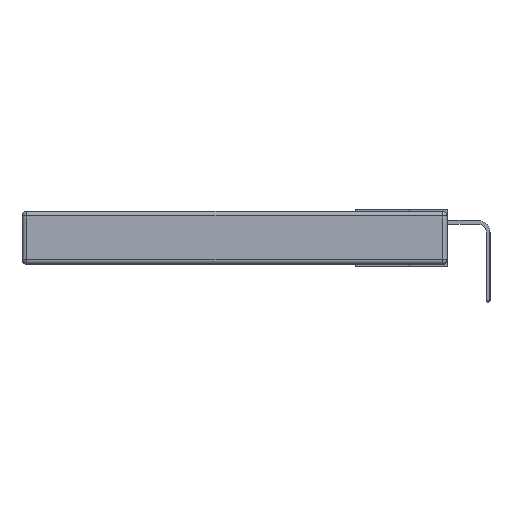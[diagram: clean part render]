
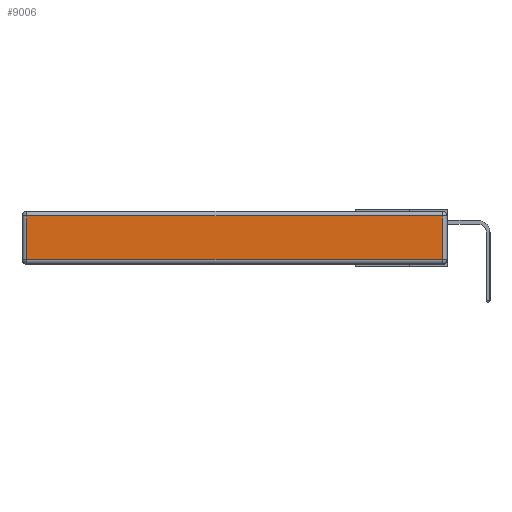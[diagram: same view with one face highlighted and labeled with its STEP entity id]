
A CAD part, left-side view. The second image highlights one B-rep face of the part: STEP entity #9006.
In plain terms, the highlighted planar face has unit normal (-1, 0, 0).
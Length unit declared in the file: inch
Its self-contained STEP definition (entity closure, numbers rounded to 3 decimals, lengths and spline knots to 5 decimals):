
#140 = PLANE ( 'NONE',  #7943 ) ;
#182 = DIRECTION ( 'NONE',  ( 0., 0., -1. ) ) ;
#898 = DIRECTION ( 'NONE',  ( 0., 1., 0. ) ) ;
#986 = VERTEX_POINT ( 'NONE', #5467 ) ;
#1932 = VECTOR ( 'NONE', #182, 39.37008 ) ;
#2548 = ORIENTED_EDGE ( 'NONE', *, *, #2623, .T. ) ;
#2623 = EDGE_CURVE ( 'NONE', #986, #3950, #15878, .T. ) ;
#2665 = CARTESIAN_POINT ( 'NONE',  ( 0., 2.72, -0.03 ) ) ;
#2863 = CARTESIAN_POINT ( 'NONE',  ( 0., 0., -0.343 ) ) ;
#3231 = FACE_OUTER_BOUND ( 'NONE', #14198, .T. ) ;
#3919 = EDGE_CURVE ( 'NONE', #7358, #15489, #17367, .T. ) ;
#3950 = VERTEX_POINT ( 'NONE', #2665 ) ;
#4594 = VECTOR ( 'NONE', #8247, 39.37008 ) ;
#5404 = EDGE_CURVE ( 'NONE', #15489, #986, #11211, .T. ) ;
#5467 = CARTESIAN_POINT ( 'NONE',  ( 0., 0.03, -0.03 ) ) ;
#6390 = ORIENTED_EDGE ( 'NONE', *, *, #3919, .T. ) ;
#6819 = CARTESIAN_POINT ( 'NONE',  ( 0., 0.03, -0.343 ) ) ;
#7358 = VERTEX_POINT ( 'NONE', #8239 ) ;
#7436 = DIRECTION ( 'NONE',  ( 0., 0., 1. ) ) ;
#7943 = AXIS2_PLACEMENT_3D ( 'NONE', #2863, #10199, #7436 ) ;
#8239 = CARTESIAN_POINT ( 'NONE',  ( 0., 2.72, -0.313 ) ) ;
#8247 = DIRECTION ( 'NONE',  ( 0., 0., 1. ) ) ;
#8455 = EDGE_CURVE ( 'NONE', #3950, #7358, #9628, .T. ) ;
#8574 = ORIENTED_EDGE ( 'NONE', *, *, #8455, .T. ) ;
#9006 = ADVANCED_FACE ( 'NONE', ( #3231 ), #140, .T. ) ;
#9628 = LINE ( 'NONE', #12599, #1932 ) ;
#10199 = DIRECTION ( 'NONE',  ( -1., 0., 0. ) ) ;
#10873 = VECTOR ( 'NONE', #898, 39.37008 ) ;
#11076 = CARTESIAN_POINT ( 'NONE',  ( 0., 0.03, -0.313 ) ) ;
#11211 = LINE ( 'NONE', #6819, #4594 ) ;
#12599 = CARTESIAN_POINT ( 'NONE',  ( 0., 2.72, -0.343 ) ) ;
#12615 = CARTESIAN_POINT ( 'NONE',  ( 0., 0., -0.313 ) ) ;
#12730 = ORIENTED_EDGE ( 'NONE', *, *, #5404, .T. ) ;
#13374 = CARTESIAN_POINT ( 'NONE',  ( 0., 2.75, -0.03 ) ) ;
#14198 = EDGE_LOOP ( 'NONE', ( #6390, #12730, #2548, #8574 ) ) ;
#14917 = VECTOR ( 'NONE', #18111, 39.37008 ) ;
#15489 = VERTEX_POINT ( 'NONE', #11076 ) ;
#15878 = LINE ( 'NONE', #13374, #10873 ) ;
#17367 = LINE ( 'NONE', #12615, #14917 ) ;
#18111 = DIRECTION ( 'NONE',  ( 0., -1., 0. ) ) ;
